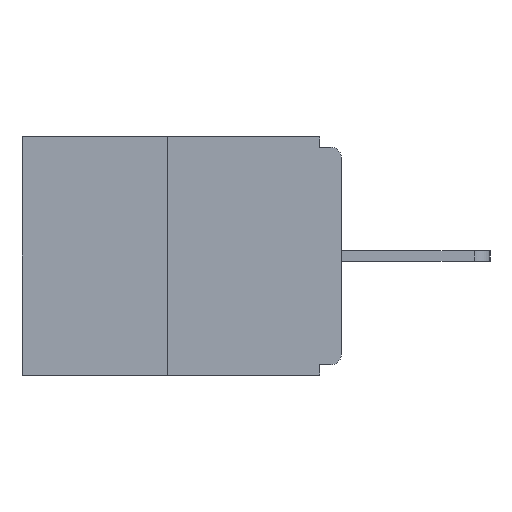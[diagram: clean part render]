
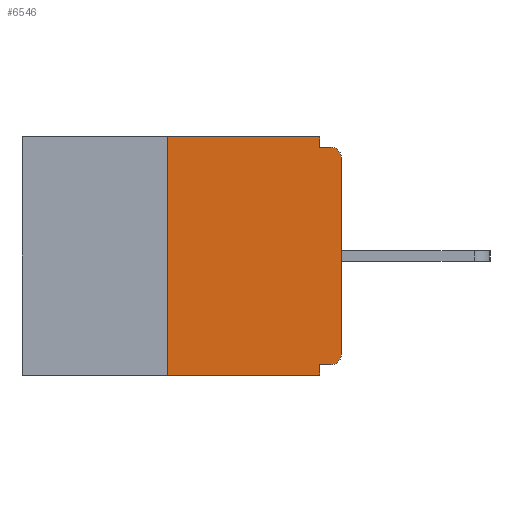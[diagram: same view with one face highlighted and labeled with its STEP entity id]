
A CAD part, left-side view. The second image highlights one B-rep face of the part: STEP entity #6546.
In plain terms, the highlighted planar face has unit normal (-1, 0, 0).
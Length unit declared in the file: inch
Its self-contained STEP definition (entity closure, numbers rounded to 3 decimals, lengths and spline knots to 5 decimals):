
#675 = EDGE_CURVE ( 'NONE', #18009, #5939, #15518, .T. ) ;
#739 = CARTESIAN_POINT ( 'NONE',  ( 0., 0.25, -0.343 ) ) ;
#785 = FACE_OUTER_BOUND ( 'NONE', #13035, .T. ) ;
#914 = CARTESIAN_POINT ( 'NONE',  ( 0., 0.015, -0.03 ) ) ;
#1384 = VERTEX_POINT ( 'NONE', #13594 ) ;
#1907 = ORIENTED_EDGE ( 'NONE', *, *, #675, .F. ) ;
#2797 = DIRECTION ( 'NONE',  ( 0., 0., -1. ) ) ;
#3469 = EDGE_CURVE ( 'NONE', #9102, #5939, #15654, .T. ) ;
#3502 = CARTESIAN_POINT ( 'NONE',  ( 0., 0.031, -0.328 ) ) ;
#3566 = ORIENTED_EDGE ( 'NONE', *, *, #17844, .F. ) ;
#3867 = CARTESIAN_POINT ( 'NONE',  ( 0., 0.46, 0. ) ) ;
#4097 = DIRECTION ( 'NONE',  ( -1., 0., 0. ) ) ;
#4519 = DIRECTION ( 'NONE',  ( 0., 0., -1. ) ) ;
#4565 = DIRECTION ( 'NONE',  ( 1., 0., 0. ) ) ;
#4631 = LINE ( 'NONE', #13586, #17492 ) ;
#4638 = PLANE ( 'NONE',  #11057 ) ;
#4993 = ORIENTED_EDGE ( 'NONE', *, *, #6293, .F. ) ;
#5254 = VECTOR ( 'NONE', #9897, 39.37008 ) ;
#5939 = VERTEX_POINT ( 'NONE', #9075 ) ;
#6293 = EDGE_CURVE ( 'NONE', #16518, #18009, #14144, .T. ) ;
#6404 = VECTOR ( 'NONE', #14124, 39.37008 ) ;
#6483 = DIRECTION ( 'NONE',  ( 0., 0., -1. ) ) ;
#6546 = ADVANCED_FACE ( 'NONE', ( #785 ), #4638, .F. ) ;
#6976 = CIRCLE ( 'NONE', #12149, 0.015 ) ;
#7013 = EDGE_CURVE ( 'NONE', #9102, #22253, #13837, .T. ) ;
#7713 = VERTEX_POINT ( 'NONE', #9455 ) ;
#7785 = ORIENTED_EDGE ( 'NONE', *, *, #16559, .T. ) ;
#8093 = CARTESIAN_POINT ( 'NONE',  ( 0., 0., -0.313 ) ) ;
#8681 = CARTESIAN_POINT ( 'NONE',  ( 0., 0., 0. ) ) ;
#8812 = EDGE_CURVE ( 'NONE', #7713, #18774, #15770, .T. ) ;
#9075 = CARTESIAN_POINT ( 'NONE',  ( 0., 0.031, -0.343 ) ) ;
#9102 = VERTEX_POINT ( 'NONE', #739 ) ;
#9176 = ORIENTED_EDGE ( 'NONE', *, *, #8812, .F. ) ;
#9440 = VECTOR ( 'NONE', #14947, 39.37008 ) ;
#9455 = CARTESIAN_POINT ( 'NONE',  ( 0., 0.031, -0.015 ) ) ;
#9724 = VECTOR ( 'NONE', #14033, 39.37008 ) ;
#9897 = DIRECTION ( 'NONE',  ( 0., -1., 0. ) ) ;
#10020 = EDGE_CURVE ( 'NONE', #17207, #13714, #21265, .T. ) ;
#11057 = AXIS2_PLACEMENT_3D ( 'NONE', #3867, #4565, #4519 ) ;
#11817 = CARTESIAN_POINT ( 'NONE',  ( 0., 0., -0.03 ) ) ;
#11874 = ORIENTED_EDGE ( 'NONE', *, *, #3469, .T. ) ;
#12149 = AXIS2_PLACEMENT_3D ( 'NONE', #914, #13349, #2797 ) ;
#12361 = CARTESIAN_POINT ( 'NONE',  ( 0., 0., -0.015 ) ) ;
#13035 = EDGE_LOOP ( 'NONE', ( #3566, #22274, #11874, #1907, #4993, #14112, #13297, #7785, #9176, #21606 ) ) ;
#13181 = EDGE_CURVE ( 'NONE', #1384, #7713, #4631, .T. ) ;
#13287 = VECTOR ( 'NONE', #19782, 39.37008 ) ;
#13297 = ORIENTED_EDGE ( 'NONE', *, *, #10020, .T. ) ;
#13349 = DIRECTION ( 'NONE',  ( -1., 0., 0. ) ) ;
#13552 = CARTESIAN_POINT ( 'NONE',  ( 0., 0.015, -0.015 ) ) ;
#13586 = CARTESIAN_POINT ( 'NONE',  ( 0., 0.031, 0. ) ) ;
#13594 = CARTESIAN_POINT ( 'NONE',  ( 0., 0.031, 0. ) ) ;
#13714 = VERTEX_POINT ( 'NONE', #11817 ) ;
#13837 = LINE ( 'NONE', #18331, #13287 ) ;
#14033 = DIRECTION ( 'NONE',  ( 0., 0., -1. ) ) ;
#14112 = ORIENTED_EDGE ( 'NONE', *, *, #20264, .T. ) ;
#14124 = DIRECTION ( 'NONE',  ( 0., -1., 0. ) ) ;
#14144 = LINE ( 'NONE', #14928, #9440 ) ;
#14289 = CIRCLE ( 'NONE', #14707, 0.015 ) ;
#14651 = CARTESIAN_POINT ( 'NONE',  ( 0., 0.015, -0.313 ) ) ;
#14707 = AXIS2_PLACEMENT_3D ( 'NONE', #14651, #4097, #16363 ) ;
#14928 = CARTESIAN_POINT ( 'NONE',  ( 0., 0., -0.328 ) ) ;
#14947 = DIRECTION ( 'NONE',  ( 0., 1., 0. ) ) ;
#15285 = CARTESIAN_POINT ( 'NONE',  ( 0., 0.46, 0. ) ) ;
#15398 = CARTESIAN_POINT ( 'NONE',  ( 0., 0.46, -0.343 ) ) ;
#15518 = LINE ( 'NONE', #18460, #9724 ) ;
#15654 = LINE ( 'NONE', #15398, #19096 ) ;
#15770 = LINE ( 'NONE', #12361, #6404 ) ;
#15815 = DIRECTION ( 'NONE',  ( 0., -1., 0. ) ) ;
#16363 = DIRECTION ( 'NONE',  ( 0., 0., -1. ) ) ;
#16518 = VERTEX_POINT ( 'NONE', #20101 ) ;
#16559 = EDGE_CURVE ( 'NONE', #13714, #18774, #6976, .T. ) ;
#17207 = VERTEX_POINT ( 'NONE', #8093 ) ;
#17492 = VECTOR ( 'NONE', #6483, 39.37008 ) ;
#17844 = EDGE_CURVE ( 'NONE', #22253, #1384, #19179, .T. ) ;
#18009 = VERTEX_POINT ( 'NONE', #3502 ) ;
#18331 = CARTESIAN_POINT ( 'NONE',  ( 0., 0.25, 0. ) ) ;
#18460 = CARTESIAN_POINT ( 'NONE',  ( 0., 0.031, -0.343 ) ) ;
#18774 = VERTEX_POINT ( 'NONE', #13552 ) ;
#19096 = VECTOR ( 'NONE', #15815, 39.37008 ) ;
#19179 = LINE ( 'NONE', #15285, #5254 ) ;
#19661 = CARTESIAN_POINT ( 'NONE',  ( 0., 0.25, 0. ) ) ;
#19782 = DIRECTION ( 'NONE',  ( 0., 0., 1. ) ) ;
#20101 = CARTESIAN_POINT ( 'NONE',  ( 0., 0.015, -0.328 ) ) ;
#20264 = EDGE_CURVE ( 'NONE', #16518, #17207, #14289, .T. ) ;
#20759 = VECTOR ( 'NONE', #22444, 39.37008 ) ;
#21265 = LINE ( 'NONE', #8681, #20759 ) ;
#21606 = ORIENTED_EDGE ( 'NONE', *, *, #13181, .F. ) ;
#22253 = VERTEX_POINT ( 'NONE', #19661 ) ;
#22274 = ORIENTED_EDGE ( 'NONE', *, *, #7013, .F. ) ;
#22444 = DIRECTION ( 'NONE',  ( 0., 0., 1. ) ) ;
